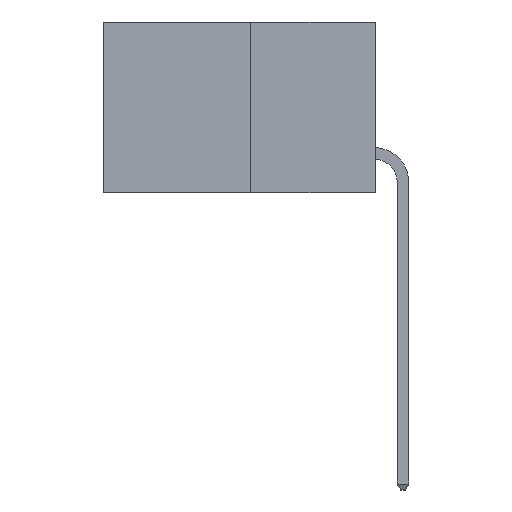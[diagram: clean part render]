
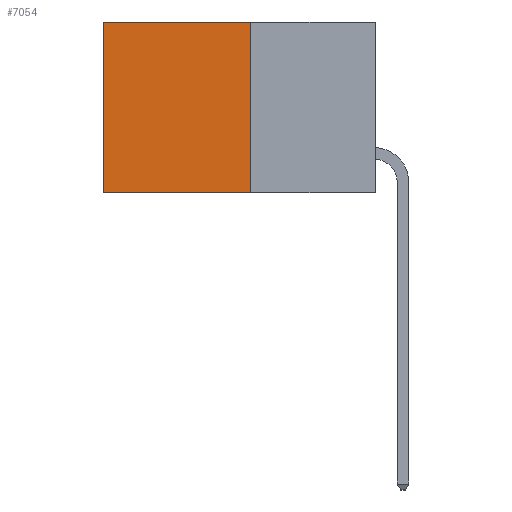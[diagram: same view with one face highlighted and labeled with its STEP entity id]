
A CAD part, left-side view. The second image highlights one B-rep face of the part: STEP entity #7054.
In plain terms, the highlighted planar face has unit normal (-1, 0, 0).
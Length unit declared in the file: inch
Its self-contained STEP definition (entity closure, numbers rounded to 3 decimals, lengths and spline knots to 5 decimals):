
#12 = CARTESIAN_POINT ( 'NONE',  ( 0.277, 0.59, -0.37 ) ) ;
#31 = DIRECTION ( 'NONE',  ( 0., 0., -1. ) ) ;
#290 = CARTESIAN_POINT ( 'NONE',  ( 0.277, 0.27, 0. ) ) ;
#815 = LINE ( 'NONE', #12894, #11701 ) ;
#1134 = LINE ( 'NONE', #10038, #6550 ) ;
#1825 = EDGE_CURVE ( 'NONE', #4328, #13038, #9947, .T. ) ;
#1842 = VERTEX_POINT ( 'NONE', #2392 ) ;
#2392 = CARTESIAN_POINT ( 'NONE',  ( 0.277, 0.27, -0.37 ) ) ;
#2420 = AXIS2_PLACEMENT_3D ( 'NONE', #9129, #8621, #11128 ) ;
#3067 = VERTEX_POINT ( 'NONE', #8572 ) ;
#4328 = VERTEX_POINT ( 'NONE', #290 ) ;
#6550 = VECTOR ( 'NONE', #7432, 39.37008 ) ;
#6954 = EDGE_CURVE ( 'NONE', #4328, #1842, #1134, .T. ) ;
#7054 = ADVANCED_FACE ( 'NONE', ( #13402 ), #9662, .F. ) ;
#7189 = VECTOR ( 'NONE', #11089, 39.37008 ) ;
#7432 = DIRECTION ( 'NONE',  ( 0., 0., -1. ) ) ;
#8572 = CARTESIAN_POINT ( 'NONE',  ( 0.277, 0.59, -0.37 ) ) ;
#8621 = DIRECTION ( 'NONE',  ( 1., 0., 0. ) ) ;
#8794 = LINE ( 'NONE', #12, #13527 ) ;
#9129 = CARTESIAN_POINT ( 'NONE',  ( 0.277, 0.27, -0.37 ) ) ;
#9347 = ORIENTED_EDGE ( 'NONE', *, *, #11319, .T. ) ;
#9357 = EDGE_CURVE ( 'NONE', #1842, #3067, #815, .T. ) ;
#9662 = PLANE ( 'NONE',  #2420 ) ;
#9947 = LINE ( 'NONE', #13429, #7189 ) ;
#10038 = CARTESIAN_POINT ( 'NONE',  ( 0.277, 0.27, -0.37 ) ) ;
#10203 = ORIENTED_EDGE ( 'NONE', *, *, #1825, .T. ) ;
#10264 = ORIENTED_EDGE ( 'NONE', *, *, #6954, .F. ) ;
#10699 = ORIENTED_EDGE ( 'NONE', *, *, #9357, .F. ) ;
#10822 = CARTESIAN_POINT ( 'NONE',  ( 0.277, 0.59, 0. ) ) ;
#11089 = DIRECTION ( 'NONE',  ( 0., 1., 0. ) ) ;
#11128 = DIRECTION ( 'NONE',  ( 0., 0., -1. ) ) ;
#11319 = EDGE_CURVE ( 'NONE', #13038, #3067, #8794, .T. ) ;
#11701 = VECTOR ( 'NONE', #12808, 39.37008 ) ;
#12808 = DIRECTION ( 'NONE',  ( 0., 1., 0. ) ) ;
#12894 = CARTESIAN_POINT ( 'NONE',  ( 0.277, 0.27, -0.37 ) ) ;
#13038 = VERTEX_POINT ( 'NONE', #10822 ) ;
#13402 = FACE_OUTER_BOUND ( 'NONE', #13487, .T. ) ;
#13429 = CARTESIAN_POINT ( 'NONE',  ( 0.277, 0.27, 0. ) ) ;
#13487 = EDGE_LOOP ( 'NONE', ( #9347, #10699, #10264, #10203 ) ) ;
#13527 = VECTOR ( 'NONE', #31, 39.37008 ) ;
